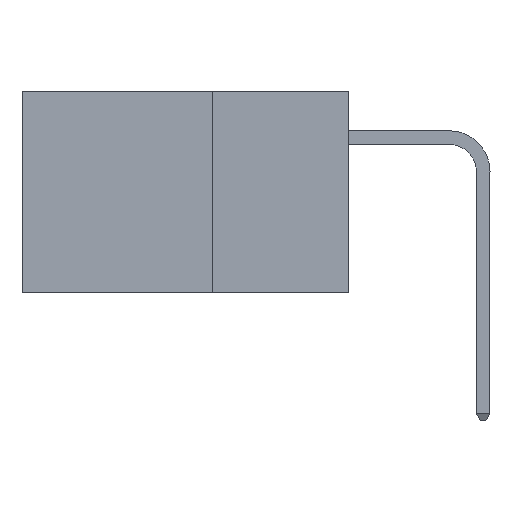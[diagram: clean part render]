
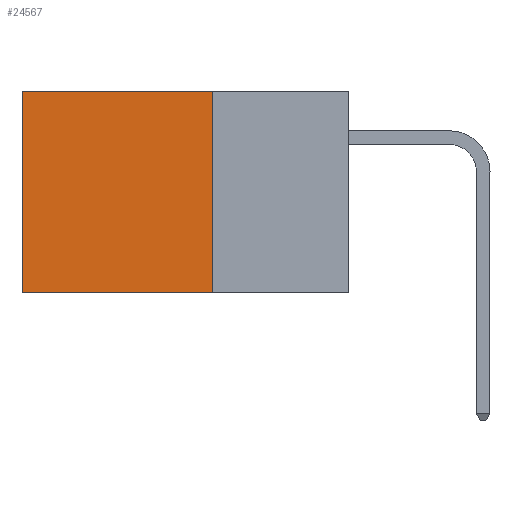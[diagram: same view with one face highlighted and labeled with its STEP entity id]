
A CAD part, left-side view. The second image highlights one B-rep face of the part: STEP entity #24567.
In plain terms, the highlighted planar face has unit normal (-1, 0, 0).
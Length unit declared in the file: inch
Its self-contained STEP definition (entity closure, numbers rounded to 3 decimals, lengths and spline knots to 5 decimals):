
#1288 = EDGE_CURVE ( 'NONE', #24268, #26399, #3414, .T. ) ;
#1403 = VECTOR ( 'NONE', #8783, 39.37008 ) ;
#2094 = ORIENTED_EDGE ( 'NONE', *, *, #1288, .T. ) ;
#2463 = VECTOR ( 'NONE', #27824, 39.37008 ) ;
#3414 = LINE ( 'NONE', #3493, #14460 ) ;
#3493 = CARTESIAN_POINT ( 'NONE',  ( 0.2875, 0.25, 0. ) ) ;
#3796 = EDGE_LOOP ( 'NONE', ( #7282, #4454, #10208, #2094 ) ) ;
#4454 = ORIENTED_EDGE ( 'NONE', *, *, #9371, .F. ) ;
#4958 = CARTESIAN_POINT ( 'NONE',  ( 0.2875, 0.25, 0. ) ) ;
#5638 = DIRECTION ( 'NONE',  ( 0., 1., 0. ) ) ;
#7018 = CARTESIAN_POINT ( 'NONE',  ( 0.2875, 0.25, 0. ) ) ;
#7282 = ORIENTED_EDGE ( 'NONE', *, *, #28381, .T. ) ;
#8246 = VECTOR ( 'NONE', #17999, 39.37008 ) ;
#8254 = VERTEX_POINT ( 'NONE', #18872 ) ;
#8448 = PLANE ( 'NONE',  #22366 ) ;
#8783 = DIRECTION ( 'NONE',  ( 0., 0., -1. ) ) ;
#9255 = CARTESIAN_POINT ( 'NONE',  ( 0.2875, 0.6, -0.37 ) ) ;
#9371 = EDGE_CURVE ( 'NONE', #8254, #25237, #11829, .T. ) ;
#9959 = CARTESIAN_POINT ( 'NONE',  ( 0.2875, 0.25, -0.37 ) ) ;
#10079 = LINE ( 'NONE', #13102, #1403 ) ;
#10208 = ORIENTED_EDGE ( 'NONE', *, *, #11489, .F. ) ;
#11489 = EDGE_CURVE ( 'NONE', #24268, #8254, #14113, .T. ) ;
#11804 = FACE_OUTER_BOUND ( 'NONE', #3796, .T. ) ;
#11829 = LINE ( 'NONE', #9959, #2463 ) ;
#12886 = DIRECTION ( 'NONE',  ( 1., 0., 0. ) ) ;
#13102 = CARTESIAN_POINT ( 'NONE',  ( 0.2875, 0.6, 0. ) ) ;
#13161 = DIRECTION ( 'NONE',  ( 0., 0., -1. ) ) ;
#14113 = LINE ( 'NONE', #4958, #8246 ) ;
#14460 = VECTOR ( 'NONE', #5638, 39.37008 ) ;
#17999 = DIRECTION ( 'NONE',  ( 0., 0., -1. ) ) ;
#18872 = CARTESIAN_POINT ( 'NONE',  ( 0.2875, 0.25, -0.37 ) ) ;
#22366 = AXIS2_PLACEMENT_3D ( 'NONE', #26088, #12886, #13161 ) ;
#24268 = VERTEX_POINT ( 'NONE', #7018 ) ;
#24567 = ADVANCED_FACE ( 'NONE', ( #11804 ), #8448, .F. ) ;
#25237 = VERTEX_POINT ( 'NONE', #9255 ) ;
#26088 = CARTESIAN_POINT ( 'NONE',  ( 0.2875, 0.25, 0. ) ) ;
#26399 = VERTEX_POINT ( 'NONE', #27158 ) ;
#27158 = CARTESIAN_POINT ( 'NONE',  ( 0.2875, 0.6, 0. ) ) ;
#27824 = DIRECTION ( 'NONE',  ( 0., 1., 0. ) ) ;
#28381 = EDGE_CURVE ( 'NONE', #26399, #25237, #10079, .T. ) ;
